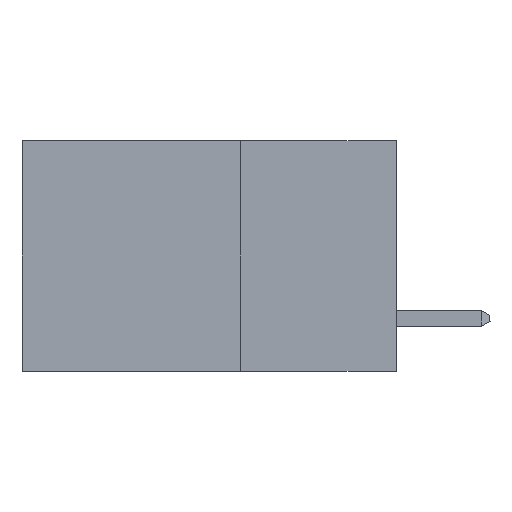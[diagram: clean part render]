
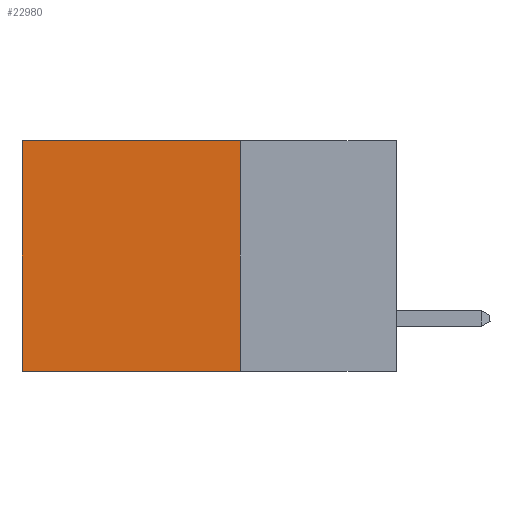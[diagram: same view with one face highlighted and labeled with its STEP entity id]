
A CAD part, left-side view. The second image highlights one B-rep face of the part: STEP entity #22980.
In plain terms, the highlighted planar face has unit normal (-1, 0, 0).
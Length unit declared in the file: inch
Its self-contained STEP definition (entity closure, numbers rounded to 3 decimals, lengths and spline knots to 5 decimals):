
#2085 = CARTESIAN_POINT ( 'NONE',  ( 0.298, 0.25, 0. ) ) ;
#2785 = CARTESIAN_POINT ( 'NONE',  ( 0.298, 0.6, -0.37 ) ) ;
#3593 = PLANE ( 'NONE',  #21500 ) ;
#4751 = DIRECTION ( 'NONE',  ( 0., 1., 0. ) ) ;
#4816 = EDGE_CURVE ( 'NONE', #14206, #20470, #18510, .T. ) ;
#5718 = DIRECTION ( 'NONE',  ( 0., 0., -1. ) ) ;
#6016 = CARTESIAN_POINT ( 'NONE',  ( 0.298, 0.6, 0. ) ) ;
#7340 = DIRECTION ( 'NONE',  ( 1., 0., 0. ) ) ;
#8089 = ORIENTED_EDGE ( 'NONE', *, *, #20936, .T. ) ;
#8121 = CARTESIAN_POINT ( 'NONE',  ( 0.298, 0.25, -0.37 ) ) ;
#8718 = LINE ( 'NONE', #2085, #21744 ) ;
#8822 = ORIENTED_EDGE ( 'NONE', *, *, #14244, .F. ) ;
#9396 = EDGE_LOOP ( 'NONE', ( #8089, #8822, #23453, #17467 ) ) ;
#10219 = VECTOR ( 'NONE', #4751, 39.37008 ) ;
#10647 = EDGE_CURVE ( 'NONE', #14206, #15398, #8718, .T. ) ;
#11927 = DIRECTION ( 'NONE',  ( 0., 1., 0. ) ) ;
#13309 = VECTOR ( 'NONE', #11927, 39.37008 ) ;
#14206 = VERTEX_POINT ( 'NONE', #16660 ) ;
#14244 = EDGE_CURVE ( 'NONE', #15398, #14893, #18625, .T. ) ;
#14893 = VERTEX_POINT ( 'NONE', #2785 ) ;
#15398 = VERTEX_POINT ( 'NONE', #20620 ) ;
#15714 = FACE_OUTER_BOUND ( 'NONE', #9396, .T. ) ;
#16058 = CARTESIAN_POINT ( 'NONE',  ( 0.298, 0.25, 0. ) ) ;
#16660 = CARTESIAN_POINT ( 'NONE',  ( 0.298, 0.25, 0. ) ) ;
#16770 = DIRECTION ( 'NONE',  ( 0., 0., -1. ) ) ;
#17467 = ORIENTED_EDGE ( 'NONE', *, *, #4816, .T. ) ;
#17559 = DIRECTION ( 'NONE',  ( 0., 0., -1. ) ) ;
#18510 = LINE ( 'NONE', #16058, #10219 ) ;
#18625 = LINE ( 'NONE', #8121, #13309 ) ;
#20470 = VERTEX_POINT ( 'NONE', #6016 ) ;
#20620 = CARTESIAN_POINT ( 'NONE',  ( 0.298, 0.25, -0.37 ) ) ;
#20936 = EDGE_CURVE ( 'NONE', #20470, #14893, #21328, .T. ) ;
#21328 = LINE ( 'NONE', #22812, #23104 ) ;
#21500 = AXIS2_PLACEMENT_3D ( 'NONE', #22563, #7340, #16770 ) ;
#21744 = VECTOR ( 'NONE', #17559, 39.37008 ) ;
#22563 = CARTESIAN_POINT ( 'NONE',  ( 0.298, 0.25, 0. ) ) ;
#22812 = CARTESIAN_POINT ( 'NONE',  ( 0.298, 0.6, 0. ) ) ;
#22980 = ADVANCED_FACE ( 'NONE', ( #15714 ), #3593, .F. ) ;
#23104 = VECTOR ( 'NONE', #5718, 39.37008 ) ;
#23453 = ORIENTED_EDGE ( 'NONE', *, *, #10647, .F. ) ;
